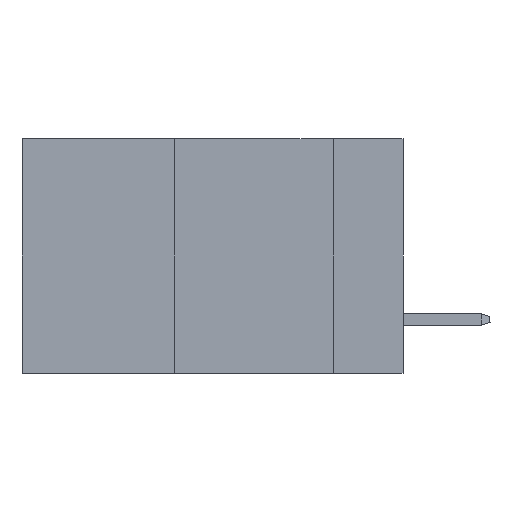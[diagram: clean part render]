
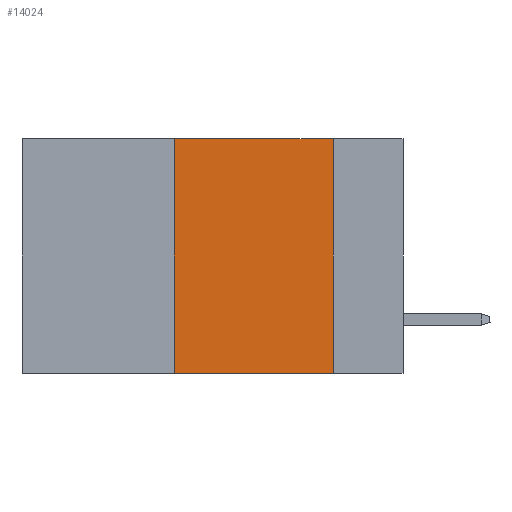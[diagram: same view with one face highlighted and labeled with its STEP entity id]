
A CAD part, left-side view. The second image highlights one B-rep face of the part: STEP entity #14024.
In plain terms, the highlighted planar face has unit normal (-1, 0, 0).
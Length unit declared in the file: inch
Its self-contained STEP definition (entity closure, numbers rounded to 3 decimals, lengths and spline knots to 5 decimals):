
#211 = CARTESIAN_POINT ( 'NONE',  ( 0., 0.36, 0. ) ) ;
#951 = ORIENTED_EDGE ( 'NONE', *, *, #6396, .T. ) ;
#1027 = CARTESIAN_POINT ( 'NONE',  ( 0., 0.11, -0.37 ) ) ;
#2949 = AXIS2_PLACEMENT_3D ( 'NONE', #13757, #8753, #16822 ) ;
#4669 = VECTOR ( 'NONE', #6215, 39.37008 ) ;
#4787 = VERTEX_POINT ( 'NONE', #24444 ) ;
#6215 = DIRECTION ( 'NONE',  ( 0., 0., 1. ) ) ;
#6396 = EDGE_CURVE ( 'NONE', #6933, #17623, #20526, .T. ) ;
#6639 = EDGE_CURVE ( 'NONE', #4787, #17623, #18786, .T. ) ;
#6933 = VERTEX_POINT ( 'NONE', #12227 ) ;
#6995 = CARTESIAN_POINT ( 'NONE',  ( 0., 0.36, 0. ) ) ;
#8377 = PLANE ( 'NONE',  #2949 ) ;
#8753 = DIRECTION ( 'NONE',  ( 1., 0., 0. ) ) ;
#8872 = EDGE_CURVE ( 'NONE', #21839, #4787, #13325, .T. ) ;
#11632 = FACE_OUTER_BOUND ( 'NONE', #25798, .T. ) ;
#12227 = CARTESIAN_POINT ( 'NONE',  ( 0., 0.36, -0.37 ) ) ;
#13325 = LINE ( 'NONE', #13530, #16780 ) ;
#13530 = CARTESIAN_POINT ( 'NONE',  ( 0., 0.6, 0. ) ) ;
#13757 = CARTESIAN_POINT ( 'NONE',  ( 0., 0.6, 0. ) ) ;
#14024 = ADVANCED_FACE ( 'NONE', ( #11632 ), #8377, .F. ) ;
#14419 = ORIENTED_EDGE ( 'NONE', *, *, #24703, .F. ) ;
#15889 = DIRECTION ( 'NONE',  ( 0., -1., 0. ) ) ;
#16480 = CARTESIAN_POINT ( 'NONE',  ( 0., 0.11, 0. ) ) ;
#16780 = VECTOR ( 'NONE', #30944, 39.37008 ) ;
#16822 = DIRECTION ( 'NONE',  ( 0., 0., -1. ) ) ;
#17623 = VERTEX_POINT ( 'NONE', #1027 ) ;
#18786 = LINE ( 'NONE', #16480, #27384 ) ;
#20526 = LINE ( 'NONE', #34354, #36014 ) ;
#20786 = LINE ( 'NONE', #211, #4669 ) ;
#21432 = ORIENTED_EDGE ( 'NONE', *, *, #8872, .F. ) ;
#21839 = VERTEX_POINT ( 'NONE', #6995 ) ;
#24444 = CARTESIAN_POINT ( 'NONE',  ( 0., 0.11, 0. ) ) ;
#24703 = EDGE_CURVE ( 'NONE', #6933, #21839, #20786, .T. ) ;
#25301 = ORIENTED_EDGE ( 'NONE', *, *, #6639, .F. ) ;
#25798 = EDGE_LOOP ( 'NONE', ( #25301, #21432, #14419, #951 ) ) ;
#27384 = VECTOR ( 'NONE', #33534, 39.37008 ) ;
#30944 = DIRECTION ( 'NONE',  ( 0., -1., 0. ) ) ;
#33534 = DIRECTION ( 'NONE',  ( 0., 0., -1. ) ) ;
#34354 = CARTESIAN_POINT ( 'NONE',  ( 0., 0.6, -0.37 ) ) ;
#36014 = VECTOR ( 'NONE', #15889, 39.37008 ) ;
